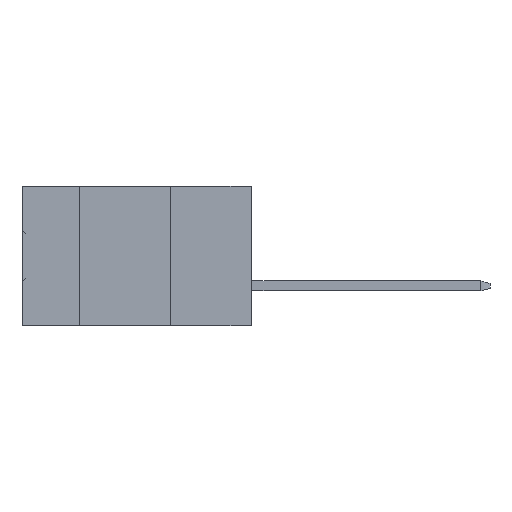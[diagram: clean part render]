
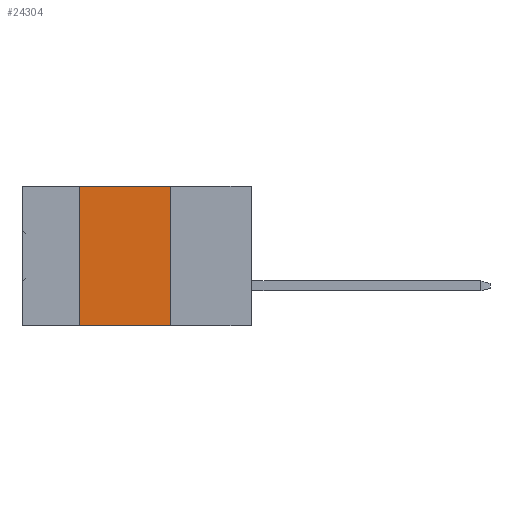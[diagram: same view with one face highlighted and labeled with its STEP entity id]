
A CAD part, left-side view. The second image highlights one B-rep face of the part: STEP entity #24304.
In plain terms, the highlighted planar face has unit normal (-1, 0, 0).
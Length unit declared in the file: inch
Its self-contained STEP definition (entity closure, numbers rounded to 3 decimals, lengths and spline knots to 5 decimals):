
#917 = LINE ( 'NONE', #10136, #13579 ) ;
#1357 = DIRECTION ( 'NONE',  ( 0., 0., 1. ) ) ;
#2204 = DIRECTION ( 'NONE',  ( 0., 0., -1. ) ) ;
#2509 = PLANE ( 'NONE',  #28699 ) ;
#4469 = FACE_OUTER_BOUND ( 'NONE', #24910, .T. ) ;
#4474 = CARTESIAN_POINT ( 'NONE',  ( 0., 0.254, 0. ) ) ;
#4618 = CARTESIAN_POINT ( 'NONE',  ( 0., 0.72, 0. ) ) ;
#4664 = EDGE_CURVE ( 'NONE', #16350, #4752, #10364, .T. ) ;
#4752 = VERTEX_POINT ( 'NONE', #6563 ) ;
#5814 = EDGE_CURVE ( 'NONE', #9054, #14132, #9670, .T. ) ;
#5820 = DIRECTION ( 'NONE',  ( 0., -1., 0. ) ) ;
#6563 = CARTESIAN_POINT ( 'NONE',  ( 0., 0.254, -0.437 ) ) ;
#6628 = ORIENTED_EDGE ( 'NONE', *, *, #6687, .F. ) ;
#6687 = EDGE_CURVE ( 'NONE', #14132, #4752, #18714, .T. ) ;
#6738 = DIRECTION ( 'NONE',  ( 1., 0., 0. ) ) ;
#7240 = ORIENTED_EDGE ( 'NONE', *, *, #5814, .F. ) ;
#9044 = CARTESIAN_POINT ( 'NONE',  ( 0., 0.254, -0.437 ) ) ;
#9054 = VERTEX_POINT ( 'NONE', #22902 ) ;
#9670 = LINE ( 'NONE', #12099, #22811 ) ;
#10136 = CARTESIAN_POINT ( 'NONE',  ( 0., 0.54, -0.437 ) ) ;
#10364 = LINE ( 'NONE', #26528, #25997 ) ;
#12099 = CARTESIAN_POINT ( 'NONE',  ( 0., 0.72, 0. ) ) ;
#13579 = VECTOR ( 'NONE', #1357, 39.37008 ) ;
#13909 = DIRECTION ( 'NONE',  ( 0., 0., -1. ) ) ;
#14132 = VERTEX_POINT ( 'NONE', #4474 ) ;
#14634 = VECTOR ( 'NONE', #13909, 39.37008 ) ;
#16350 = VERTEX_POINT ( 'NONE', #18141 ) ;
#17929 = EDGE_CURVE ( 'NONE', #16350, #9054, #917, .T. ) ;
#18021 = ORIENTED_EDGE ( 'NONE', *, *, #17929, .F. ) ;
#18141 = CARTESIAN_POINT ( 'NONE',  ( 0., 0.54, -0.437 ) ) ;
#18714 = LINE ( 'NONE', #9044, #14634 ) ;
#22811 = VECTOR ( 'NONE', #26131, 39.37008 ) ;
#22902 = CARTESIAN_POINT ( 'NONE',  ( 0., 0.54, 0. ) ) ;
#24304 = ADVANCED_FACE ( 'NONE', ( #4469 ), #2509, .F. ) ;
#24910 = EDGE_LOOP ( 'NONE', ( #6628, #7240, #18021, #26624 ) ) ;
#25997 = VECTOR ( 'NONE', #5820, 39.37008 ) ;
#26131 = DIRECTION ( 'NONE',  ( 0., -1., 0. ) ) ;
#26528 = CARTESIAN_POINT ( 'NONE',  ( 0., 0.72, -0.437 ) ) ;
#26624 = ORIENTED_EDGE ( 'NONE', *, *, #4664, .T. ) ;
#28699 = AXIS2_PLACEMENT_3D ( 'NONE', #4618, #6738, #2204 ) ;
